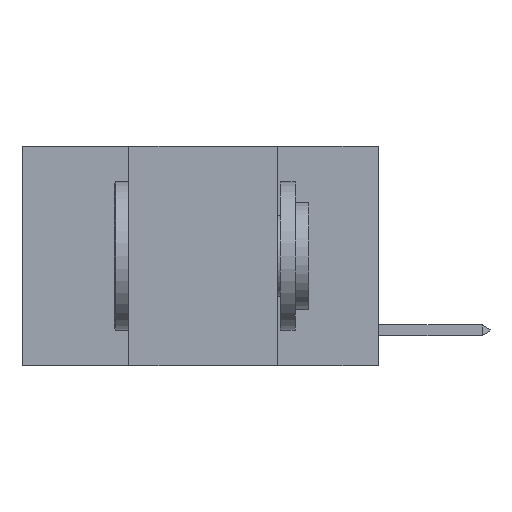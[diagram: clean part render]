
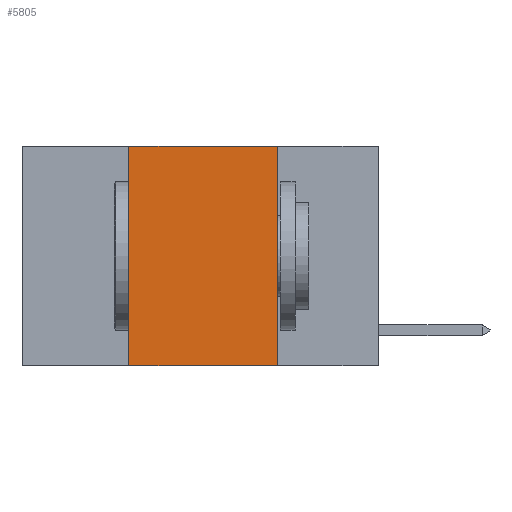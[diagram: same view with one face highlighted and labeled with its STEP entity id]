
A CAD part, left-side view. The second image highlights one B-rep face of the part: STEP entity #5805.
In plain terms, the highlighted planar face has unit normal (-1, 0, 0).
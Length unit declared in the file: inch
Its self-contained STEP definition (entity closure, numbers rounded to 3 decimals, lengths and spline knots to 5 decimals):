
#927 = VERTEX_POINT ( 'NONE', #8852 ) ;
#1193 = CARTESIAN_POINT ( 'NONE',  ( 0., 0.6, 0. ) ) ;
#1225 = DIRECTION ( 'NONE',  ( 0., -1., 0. ) ) ;
#3091 = EDGE_CURVE ( 'NONE', #4403, #15169, #5354, .T. ) ;
#3151 = EDGE_CURVE ( 'NONE', #4403, #927, #19516, .T. ) ;
#3496 = EDGE_CURVE ( 'NONE', #15169, #13731, #15082, .T. ) ;
#4403 = VERTEX_POINT ( 'NONE', #20772 ) ;
#4493 = ORIENTED_EDGE ( 'NONE', *, *, #3496, .F. ) ;
#4606 = AXIS2_PLACEMENT_3D ( 'NONE', #6667, #13082, #23511 ) ;
#5354 = LINE ( 'NONE', #19126, #19935 ) ;
#5805 = ADVANCED_FACE ( 'NONE', ( #7078 ), #19092, .F. ) ;
#6291 = ORIENTED_EDGE ( 'NONE', *, *, #14176, .F. ) ;
#6667 = CARTESIAN_POINT ( 'NONE',  ( 0., 0.6, 0. ) ) ;
#6972 = CARTESIAN_POINT ( 'NONE',  ( 0., 0.6, -0.37 ) ) ;
#7078 = FACE_OUTER_BOUND ( 'NONE', #9986, .T. ) ;
#8852 = CARTESIAN_POINT ( 'NONE',  ( 0., 0.17, -0.37 ) ) ;
#9986 = EDGE_LOOP ( 'NONE', ( #6291, #4493, #23195, #16053 ) ) ;
#10328 = CARTESIAN_POINT ( 'NONE',  ( 0., 0.42, 0. ) ) ;
#10352 = VECTOR ( 'NONE', #21876, 39.37008 ) ;
#13082 = DIRECTION ( 'NONE',  ( 1., 0., 0. ) ) ;
#13731 = VERTEX_POINT ( 'NONE', #14481 ) ;
#14176 = EDGE_CURVE ( 'NONE', #13731, #927, #19466, .T. ) ;
#14481 = CARTESIAN_POINT ( 'NONE',  ( 0., 0.17, 0. ) ) ;
#15082 = LINE ( 'NONE', #1193, #18284 ) ;
#15169 = VERTEX_POINT ( 'NONE', #10328 ) ;
#15242 = DIRECTION ( 'NONE',  ( 0., 0., 1. ) ) ;
#16053 = ORIENTED_EDGE ( 'NONE', *, *, #3151, .T. ) ;
#18284 = VECTOR ( 'NONE', #21495, 39.37008 ) ;
#19092 = PLANE ( 'NONE',  #4606 ) ;
#19126 = CARTESIAN_POINT ( 'NONE',  ( 0., 0.42, 0. ) ) ;
#19466 = LINE ( 'NONE', #21744, #10352 ) ;
#19516 = LINE ( 'NONE', #6972, #19523 ) ;
#19523 = VECTOR ( 'NONE', #1225, 39.37008 ) ;
#19935 = VECTOR ( 'NONE', #15242, 39.37008 ) ;
#20772 = CARTESIAN_POINT ( 'NONE',  ( 0., 0.42, -0.37 ) ) ;
#21495 = DIRECTION ( 'NONE',  ( 0., -1., 0. ) ) ;
#21744 = CARTESIAN_POINT ( 'NONE',  ( 0., 0.17, 0. ) ) ;
#21876 = DIRECTION ( 'NONE',  ( 0., 0., -1. ) ) ;
#23195 = ORIENTED_EDGE ( 'NONE', *, *, #3091, .F. ) ;
#23511 = DIRECTION ( 'NONE',  ( 0., 0., -1. ) ) ;
